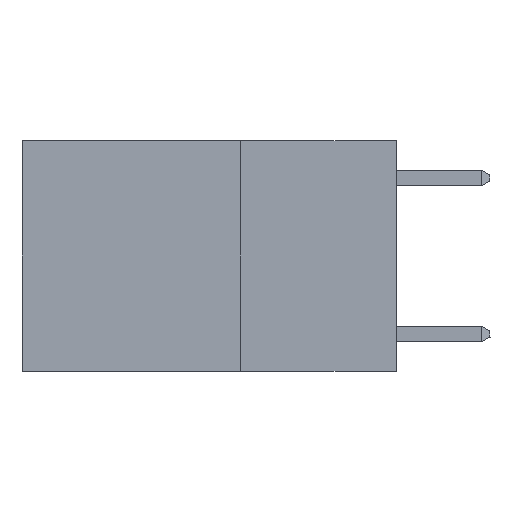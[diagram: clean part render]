
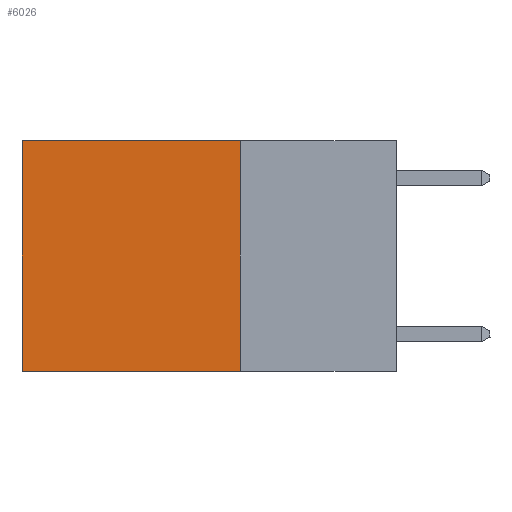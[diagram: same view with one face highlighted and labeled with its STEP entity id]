
A CAD part, left-side view. The second image highlights one B-rep face of the part: STEP entity #6026.
In plain terms, the highlighted planar face has unit normal (-1, 0, 0).
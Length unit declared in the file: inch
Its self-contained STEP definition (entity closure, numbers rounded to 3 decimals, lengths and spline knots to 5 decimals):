
#1468 = EDGE_CURVE ( 'NONE', #11670, #17324, #9486, .T. ) ;
#1472 = DIRECTION ( 'NONE',  ( 0., 1., 0. ) ) ;
#2178 = CARTESIAN_POINT ( 'NONE',  ( 0.2625, 0.25, 0. ) ) ;
#2735 = CARTESIAN_POINT ( 'NONE',  ( 0.2625, 0.25, 0. ) ) ;
#3351 = ORIENTED_EDGE ( 'NONE', *, *, #1468, .F. ) ;
#3728 = CARTESIAN_POINT ( 'NONE',  ( 0.2625, 0.25, 0. ) ) ;
#4818 = CARTESIAN_POINT ( 'NONE',  ( 0.2625, 0.6, -0.37 ) ) ;
#5355 = DIRECTION ( 'NONE',  ( 0., 0., -1. ) ) ;
#5444 = EDGE_CURVE ( 'NONE', #11670, #5602, #16112, .T. ) ;
#5602 = VERTEX_POINT ( 'NONE', #12848 ) ;
#6026 = ADVANCED_FACE ( 'NONE', ( #9782 ), #16761, .F. ) ;
#6906 = ORIENTED_EDGE ( 'NONE', *, *, #5444, .T. ) ;
#7283 = CARTESIAN_POINT ( 'NONE',  ( 0.2625, 0.25, 0. ) ) ;
#7600 = VECTOR ( 'NONE', #1472, 39.37008 ) ;
#7775 = CARTESIAN_POINT ( 'NONE',  ( 0.2625, 0.25, -0.37 ) ) ;
#8749 = EDGE_CURVE ( 'NONE', #5602, #10723, #10164, .T. ) ;
#8938 = DIRECTION ( 'NONE',  ( 1., 0., 0. ) ) ;
#9419 = VECTOR ( 'NONE', #5355, 39.37008 ) ;
#9486 = LINE ( 'NONE', #3728, #9419 ) ;
#9782 = FACE_OUTER_BOUND ( 'NONE', #14427, .T. ) ;
#9928 = VECTOR ( 'NONE', #17095, 39.37008 ) ;
#10164 = LINE ( 'NONE', #12588, #9928 ) ;
#10723 = VERTEX_POINT ( 'NONE', #4818 ) ;
#11670 = VERTEX_POINT ( 'NONE', #2178 ) ;
#11849 = ORIENTED_EDGE ( 'NONE', *, *, #19635, .F. ) ;
#11937 = LINE ( 'NONE', #12894, #7600 ) ;
#12588 = CARTESIAN_POINT ( 'NONE',  ( 0.2625, 0.6, 0. ) ) ;
#12848 = CARTESIAN_POINT ( 'NONE',  ( 0.2625, 0.6, 0. ) ) ;
#12894 = CARTESIAN_POINT ( 'NONE',  ( 0.2625, 0.25, -0.37 ) ) ;
#14427 = EDGE_LOOP ( 'NONE', ( #15638, #11849, #3351, #6906 ) ) ;
#15624 = DIRECTION ( 'NONE',  ( 0., 1., 0. ) ) ;
#15638 = ORIENTED_EDGE ( 'NONE', *, *, #8749, .T. ) ;
#15642 = AXIS2_PLACEMENT_3D ( 'NONE', #7283, #8938, #19530 ) ;
#16006 = VECTOR ( 'NONE', #15624, 39.37008 ) ;
#16112 = LINE ( 'NONE', #2735, #16006 ) ;
#16761 = PLANE ( 'NONE',  #15642 ) ;
#17095 = DIRECTION ( 'NONE',  ( 0., 0., -1. ) ) ;
#17324 = VERTEX_POINT ( 'NONE', #7775 ) ;
#19530 = DIRECTION ( 'NONE',  ( 0., 0., -1. ) ) ;
#19635 = EDGE_CURVE ( 'NONE', #17324, #10723, #11937, .T. ) ;
